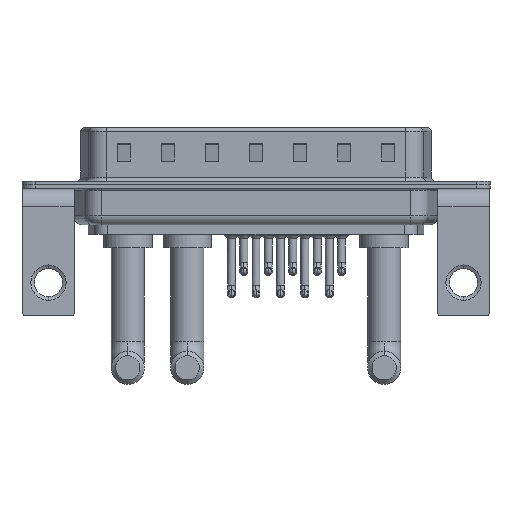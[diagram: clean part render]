
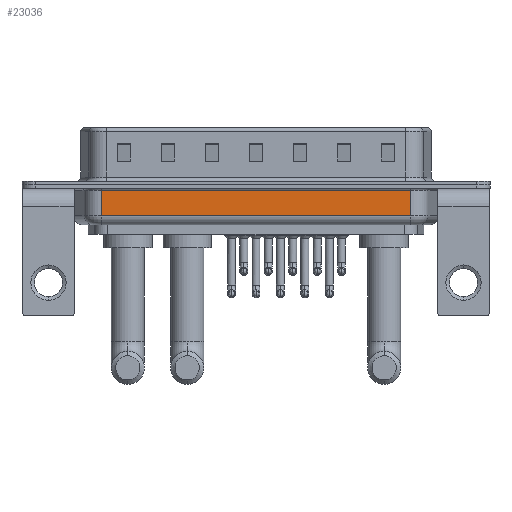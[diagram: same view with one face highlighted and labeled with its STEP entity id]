
A CAD part, front view. The second image highlights one B-rep face of the part: STEP entity #23036.
In plain terms, the highlighted planar face has unit normal (0, -1, 0).
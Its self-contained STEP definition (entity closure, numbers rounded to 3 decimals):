
#341 = LINE ( 'NONE', #22177, #10336 ) ;
#1492 = CARTESIAN_POINT ( 'NONE',  ( 6.006, -5.35, -3.5 ) ) ;
#2260 = CARTESIAN_POINT ( 'NONE',  ( 6.006, -5.35, -3.5 ) ) ;
#2569 = CARTESIAN_POINT ( 'NONE',  ( 41.044, -5.35, -3.5 ) ) ;
#2741 = CARTESIAN_POINT ( 'NONE',  ( 6.006, -5.35, -4.5 ) ) ;
#4154 = VECTOR ( 'NONE', #9791, 1000. ) ;
#4598 = DIRECTION ( 'NONE',  ( 0., 0., 1. ) ) ;
#4823 = CARTESIAN_POINT ( 'NONE',  ( 6.006, -5.35, -0.65 ) ) ;
#4842 = DIRECTION ( 'NONE',  ( 0., 1., 0. ) ) ;
#4904 = LINE ( 'NONE', #10593, #15846 ) ;
#6441 = LINE ( 'NONE', #4823, #20385 ) ;
#8123 = VERTEX_POINT ( 'NONE', #24216 ) ;
#8342 = ORIENTED_EDGE ( 'NONE', *, *, #10397, .T. ) ;
#8936 = EDGE_CURVE ( 'NONE', #21998, #12395, #4904, .T. ) ;
#9791 = DIRECTION ( 'NONE',  ( 1., 0., 0. ) ) ;
#10336 = VECTOR ( 'NONE', #22760, 1000. ) ;
#10392 = DIRECTION ( 'NONE',  ( -1., 0., 0. ) ) ;
#10397 = EDGE_CURVE ( 'NONE', #17751, #8123, #341, .T. ) ;
#10593 = CARTESIAN_POINT ( 'NONE',  ( 6.006, -5.35, -4.5 ) ) ;
#11770 = LINE ( 'NONE', #2260, #4154 ) ;
#12395 = VERTEX_POINT ( 'NONE', #19245 ) ;
#12764 = ORIENTED_EDGE ( 'NONE', *, *, #8936, .F. ) ;
#14422 = ORIENTED_EDGE ( 'NONE', *, *, #18636, .T. ) ;
#15441 = EDGE_CURVE ( 'NONE', #21998, #17751, #11770, .T. ) ;
#15846 = VECTOR ( 'NONE', #22146, 1000. ) ;
#17751 = VERTEX_POINT ( 'NONE', #2569 ) ;
#17806 = FACE_OUTER_BOUND ( 'NONE', #22934, .T. ) ;
#18636 = EDGE_CURVE ( 'NONE', #8123, #12395, #6441, .T. ) ;
#19245 = CARTESIAN_POINT ( 'NONE',  ( 6.006, -5.35, -0.65 ) ) ;
#20385 = VECTOR ( 'NONE', #10392, 1000. ) ;
#21998 = VERTEX_POINT ( 'NONE', #1492 ) ;
#22071 = AXIS2_PLACEMENT_3D ( 'NONE', #2741, #4842, #4598 ) ;
#22146 = DIRECTION ( 'NONE',  ( 0., 0., 1. ) ) ;
#22177 = CARTESIAN_POINT ( 'NONE',  ( 41.044, -5.35, -4.5 ) ) ;
#22686 = ORIENTED_EDGE ( 'NONE', *, *, #15441, .T. ) ;
#22760 = DIRECTION ( 'NONE',  ( 0., 0., 1. ) ) ;
#22934 = EDGE_LOOP ( 'NONE', ( #12764, #22686, #8342, #14422 ) ) ;
#23036 = ADVANCED_FACE ( 'NONE', ( #17806 ), #23702, .F. ) ;
#23702 = PLANE ( 'NONE',  #22071 ) ;
#24216 = CARTESIAN_POINT ( 'NONE',  ( 41.044, -5.35, -0.65 ) ) ;
